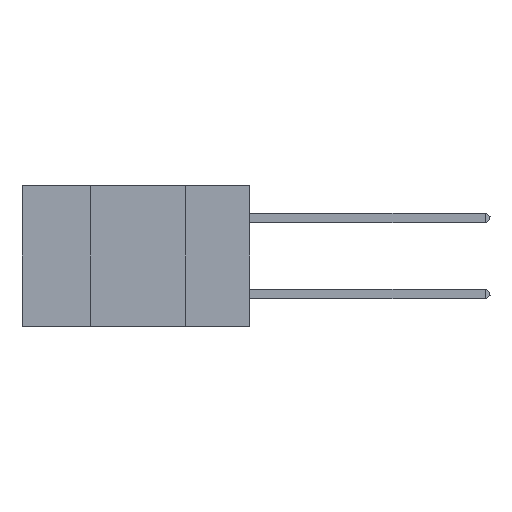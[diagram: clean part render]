
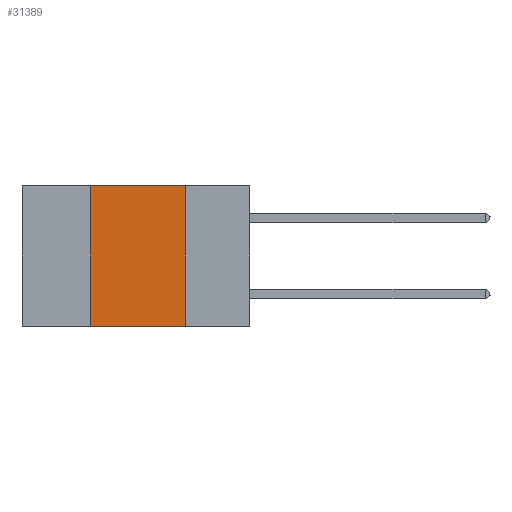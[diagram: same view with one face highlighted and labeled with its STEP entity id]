
A CAD part, left-side view. The second image highlights one B-rep face of the part: STEP entity #31389.
In plain terms, the highlighted planar face has unit normal (-1, 0, 0).
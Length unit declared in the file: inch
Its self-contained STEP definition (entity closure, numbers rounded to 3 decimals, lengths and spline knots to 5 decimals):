
#350 = CARTESIAN_POINT ( 'NONE',  ( 0., 0.42, 0. ) ) ;
#1035 = ORIENTED_EDGE ( 'NONE', *, *, #11950, .F. ) ;
#1542 = CARTESIAN_POINT ( 'NONE',  ( 0., 0.6, 0. ) ) ;
#3858 = FACE_OUTER_BOUND ( 'NONE', #29794, .T. ) ;
#3886 = EDGE_CURVE ( 'NONE', #13302, #31205, #18716, .T. ) ;
#4154 = VECTOR ( 'NONE', #4655, 39.37008 ) ;
#4273 = VECTOR ( 'NONE', #28061, 39.37008 ) ;
#4655 = DIRECTION ( 'NONE',  ( 0., -1., 0. ) ) ;
#6881 = DIRECTION ( 'NONE',  ( 1., 0., 0. ) ) ;
#8000 = DIRECTION ( 'NONE',  ( 0., -1., 0. ) ) ;
#8318 = CARTESIAN_POINT ( 'NONE',  ( 0., 0.17, -0.37 ) ) ;
#8872 = EDGE_CURVE ( 'NONE', #13302, #27322, #19564, .T. ) ;
#10971 = DIRECTION ( 'NONE',  ( 0., 0., 1. ) ) ;
#11950 = EDGE_CURVE ( 'NONE', #31205, #20573, #29315, .T. ) ;
#12600 = CARTESIAN_POINT ( 'NONE',  ( 0., 0.17, 0. ) ) ;
#13302 = VERTEX_POINT ( 'NONE', #31623 ) ;
#14211 = DIRECTION ( 'NONE',  ( 0., 0., -1. ) ) ;
#14573 = CARTESIAN_POINT ( 'NONE',  ( 0., 0.6, -0.37 ) ) ;
#15021 = LINE ( 'NONE', #12600, #4273 ) ;
#17151 = ORIENTED_EDGE ( 'NONE', *, *, #21984, .F. ) ;
#18716 = LINE ( 'NONE', #350, #30996 ) ;
#18793 = CARTESIAN_POINT ( 'NONE',  ( 0., 0.17, 0. ) ) ;
#19254 = PLANE ( 'NONE',  #20871 ) ;
#19564 = LINE ( 'NONE', #14573, #4154 ) ;
#20573 = VERTEX_POINT ( 'NONE', #18793 ) ;
#20871 = AXIS2_PLACEMENT_3D ( 'NONE', #26773, #6881, #14211 ) ;
#21984 = EDGE_CURVE ( 'NONE', #20573, #27322, #15021, .T. ) ;
#22026 = VECTOR ( 'NONE', #8000, 39.37008 ) ;
#26030 = CARTESIAN_POINT ( 'NONE',  ( 0., 0.42, 0. ) ) ;
#26773 = CARTESIAN_POINT ( 'NONE',  ( 0., 0.6, 0. ) ) ;
#27322 = VERTEX_POINT ( 'NONE', #8318 ) ;
#28061 = DIRECTION ( 'NONE',  ( 0., 0., -1. ) ) ;
#28812 = ORIENTED_EDGE ( 'NONE', *, *, #8872, .T. ) ;
#29172 = ORIENTED_EDGE ( 'NONE', *, *, #3886, .F. ) ;
#29315 = LINE ( 'NONE', #1542, #22026 ) ;
#29794 = EDGE_LOOP ( 'NONE', ( #17151, #1035, #29172, #28812 ) ) ;
#30996 = VECTOR ( 'NONE', #10971, 39.37008 ) ;
#31205 = VERTEX_POINT ( 'NONE', #26030 ) ;
#31389 = ADVANCED_FACE ( 'NONE', ( #3858 ), #19254, .F. ) ;
#31623 = CARTESIAN_POINT ( 'NONE',  ( 0., 0.42, -0.37 ) ) ;
